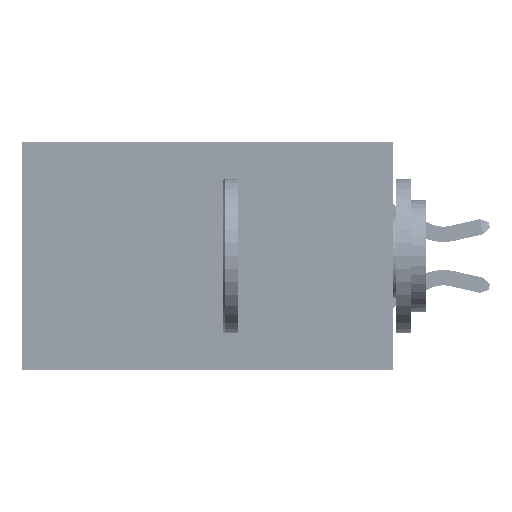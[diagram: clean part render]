
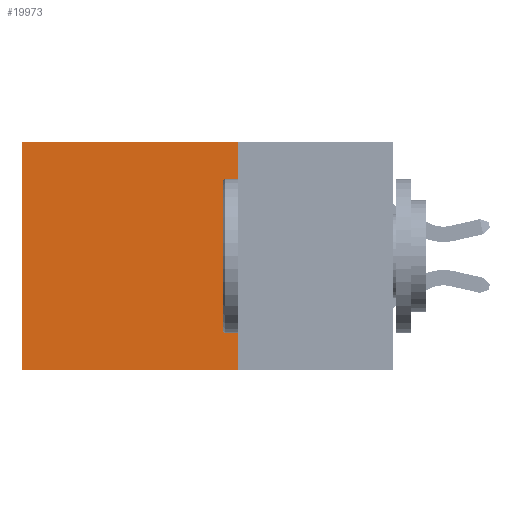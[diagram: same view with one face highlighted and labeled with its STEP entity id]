
A CAD part, left-side view. The second image highlights one B-rep face of the part: STEP entity #19973.
In plain terms, the highlighted planar face has unit normal (-1, 0, 0).
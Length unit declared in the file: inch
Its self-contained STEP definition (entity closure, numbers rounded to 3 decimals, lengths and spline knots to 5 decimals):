
#3232 = ORIENTED_EDGE ( 'NONE', *, *, #14515, .T. ) ;
#3417 = ORIENTED_EDGE ( 'NONE', *, *, #14797, .T. ) ;
#6052 = CARTESIAN_POINT ( 'NONE',  ( 0.2875, 0.25, 0. ) ) ;
#6171 = LINE ( 'NONE', #29530, #40399 ) ;
#7307 = FACE_OUTER_BOUND ( 'NONE', #41601, .T. ) ;
#7543 = CARTESIAN_POINT ( 'NONE',  ( 0.2875, 0.25, 0. ) ) ;
#7579 = CARTESIAN_POINT ( 'NONE',  ( 0.2875, 0.25, 0. ) ) ;
#9849 = CARTESIAN_POINT ( 'NONE',  ( 0.2875, 0.6, -0.37 ) ) ;
#9959 = CARTESIAN_POINT ( 'NONE',  ( 0.2875, 0.6, 0. ) ) ;
#10800 = CARTESIAN_POINT ( 'NONE',  ( 0.2875, 0.25, 0. ) ) ;
#11001 = DIRECTION ( 'NONE',  ( 0., 1., 0. ) ) ;
#13950 = DIRECTION ( 'NONE',  ( 1., 0., 0. ) ) ;
#14515 = EDGE_CURVE ( 'NONE', #16571, #38593, #29135, .T. ) ;
#14797 = EDGE_CURVE ( 'NONE', #21668, #16571, #16332, .T. ) ;
#16332 = LINE ( 'NONE', #7543, #38761 ) ;
#16571 = VERTEX_POINT ( 'NONE', #34226 ) ;
#19973 = ADVANCED_FACE ( 'NONE', ( #7307 ), #24107, .F. ) ;
#21361 = EDGE_CURVE ( 'NONE', #21668, #35513, #23728, .T. ) ;
#21668 = VERTEX_POINT ( 'NONE', #6052 ) ;
#22381 = DIRECTION ( 'NONE',  ( 0., 1., 0. ) ) ;
#23258 = AXIS2_PLACEMENT_3D ( 'NONE', #10800, #13950, #37853 ) ;
#23728 = LINE ( 'NONE', #7579, #34957 ) ;
#24107 = PLANE ( 'NONE',  #23258 ) ;
#26298 = EDGE_CURVE ( 'NONE', #35513, #38593, #6171, .T. ) ;
#29135 = LINE ( 'NONE', #9959, #37167 ) ;
#29530 = CARTESIAN_POINT ( 'NONE',  ( 0.2875, 0.25, -0.37 ) ) ;
#31495 = DIRECTION ( 'NONE',  ( 0., 0., -1. ) ) ;
#33856 = DIRECTION ( 'NONE',  ( 0., 0., -1. ) ) ;
#34003 = ORIENTED_EDGE ( 'NONE', *, *, #21361, .F. ) ;
#34152 = CARTESIAN_POINT ( 'NONE',  ( 0.2875, 0.25, -0.37 ) ) ;
#34226 = CARTESIAN_POINT ( 'NONE',  ( 0.2875, 0.6, 0. ) ) ;
#34957 = VECTOR ( 'NONE', #31495, 39.37008 ) ;
#35513 = VERTEX_POINT ( 'NONE', #34152 ) ;
#35766 = ORIENTED_EDGE ( 'NONE', *, *, #26298, .F. ) ;
#37167 = VECTOR ( 'NONE', #33856, 39.37008 ) ;
#37853 = DIRECTION ( 'NONE',  ( 0., 0., -1. ) ) ;
#38593 = VERTEX_POINT ( 'NONE', #9849 ) ;
#38761 = VECTOR ( 'NONE', #11001, 39.37008 ) ;
#40399 = VECTOR ( 'NONE', #22381, 39.37008 ) ;
#41601 = EDGE_LOOP ( 'NONE', ( #3232, #35766, #34003, #3417 ) ) ;
